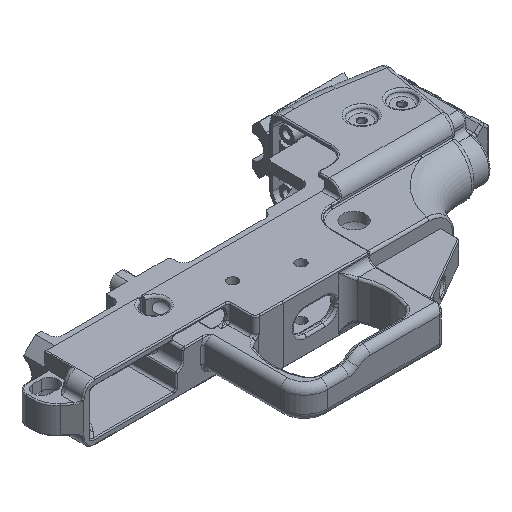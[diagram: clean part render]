
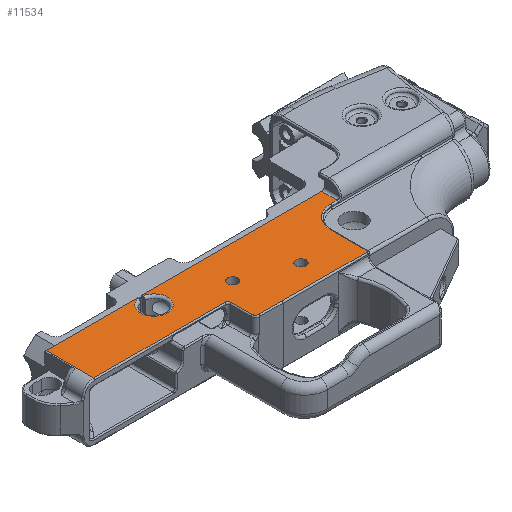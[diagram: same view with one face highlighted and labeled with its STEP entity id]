
A CAD part, isometric view. The second image highlights one B-rep face of the part: STEP entity #11534.
In plain terms, the highlighted face is planar.
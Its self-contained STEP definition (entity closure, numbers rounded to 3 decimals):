
#192=FACE_BOUND('',#2251,.T.);
#193=FACE_BOUND('',#2252,.T.);
#549=CIRCLE('',#12264,2.175);
#551=CIRCLE('',#12267,2.175);
#599=CIRCLE('',#12346,5.875);
#602=CIRCLE('',#12353,0.5);
#605=CIRCLE('',#12357,0.5);
#609=CIRCLE('',#12363,1.5);
#610=CIRCLE('',#12364,1.5);
#611=CIRCLE('',#12365,0.5);
#612=CIRCLE('',#12366,9.5);
#1534=FACE_OUTER_BOUND('',#2250,.T.);
#2250=EDGE_LOOP('',(#7943,#7944,#7945,#7946,#7947,#7948,#7949,#7950,#7951,
#7952,#7953,#7954,#7955,#7956,#7957,#7958,#7959,#7960,#7961));
#2251=EDGE_LOOP('',(#7962));
#2252=EDGE_LOOP('',(#7963));
#2956=LINE('',#17332,#3840);
#2996=LINE('',#17995,#3880);
#3036=LINE('',#18155,#3920);
#3038=LINE('',#18324,#3922);
#3046=LINE('',#18387,#3930);
#3047=LINE('',#18389,#3931);
#3048=LINE('',#18393,#3932);
#3049=LINE('',#18397,#3933);
#3050=LINE('',#18399,#3934);
#3051=LINE('',#18403,#3935);
#3052=LINE('',#18407,#3936);
#3053=LINE('',#18408,#3937);
#3840=VECTOR('',#13659,10.);
#3880=VECTOR('',#13839,10.);
#3920=VECTOR('',#13969,10.);
#3922=VECTOR('',#13977,10.);
#3930=VECTOR('',#14007,39.75);
#3931=VECTOR('',#14008,10.);
#3932=VECTOR('',#14011,10.);
#3933=VECTOR('',#14014,10.);
#3934=VECTOR('',#14015,10.);
#3935=VECTOR('',#14018,10.);
#3936=VECTOR('',#14021,10.);
#3937=VECTOR('',#14022,10.);
#4730=VERTEX_POINT('',#17329);
#4731=VERTEX_POINT('',#17331);
#4769=VERTEX_POINT('',#17462);
#4771=VERTEX_POINT('',#17468);
#4810=VERTEX_POINT('',#17992);
#4811=VERTEX_POINT('',#17994);
#4861=VERTEX_POINT('',#18122);
#4862=VERTEX_POINT('',#18133);
#4866=VERTEX_POINT('',#18153);
#4873=VERTEX_POINT('',#18323);
#4878=VERTEX_POINT('',#18338);
#4884=VERTEX_POINT('',#18388);
#4885=VERTEX_POINT('',#18390);
#4886=VERTEX_POINT('',#18392);
#4887=VERTEX_POINT('',#18394);
#4888=VERTEX_POINT('',#18396);
#4889=VERTEX_POINT('',#18398);
#4890=VERTEX_POINT('',#18400);
#4891=VERTEX_POINT('',#18402);
#4892=VERTEX_POINT('',#18404);
#4893=VERTEX_POINT('',#18406);
#5839=EDGE_CURVE('',#4730,#4731,#2956,.T.);
#5887=EDGE_CURVE('',#4769,#4769,#549,.T.);
#5890=EDGE_CURVE('',#4771,#4771,#551,.T.);
#5945=EDGE_CURVE('',#4810,#4811,#2996,.T.);
#6009=EDGE_CURVE('',#4861,#4862,#599,.T.);
#6016=EDGE_CURVE('',#4861,#4866,#3036,.T.);
#6025=EDGE_CURVE('',#4873,#4862,#3038,.T.);
#6029=EDGE_CURVE('',#4730,#4873,#602,.T.);
#6033=EDGE_CURVE('',#4866,#4878,#605,.T.);
#6041=EDGE_CURVE('',#4811,#4878,#3046,.T.);
#6042=EDGE_CURVE('',#4884,#4810,#3047,.T.);
#6043=EDGE_CURVE('',#4885,#4884,#609,.T.);
#6044=EDGE_CURVE('',#4886,#4885,#3048,.T.);
#6045=EDGE_CURVE('',#4887,#4886,#610,.T.);
#6046=EDGE_CURVE('',#4888,#4887,#3049,.T.);
#6047=EDGE_CURVE('',#4889,#4888,#3050,.T.);
#6048=EDGE_CURVE('',#4890,#4889,#611,.T.);
#6049=EDGE_CURVE('',#4891,#4890,#3051,.T.);
#6050=EDGE_CURVE('',#4892,#4891,#612,.T.);
#6051=EDGE_CURVE('',#4893,#4892,#3052,.T.);
#6052=EDGE_CURVE('',#4731,#4893,#3053,.T.);
#7943=ORIENTED_EDGE('',*,*,#6041,.F.);
#7944=ORIENTED_EDGE('',*,*,#5945,.F.);
#7945=ORIENTED_EDGE('',*,*,#6042,.F.);
#7946=ORIENTED_EDGE('',*,*,#6043,.F.);
#7947=ORIENTED_EDGE('',*,*,#6044,.F.);
#7948=ORIENTED_EDGE('',*,*,#6045,.F.);
#7949=ORIENTED_EDGE('',*,*,#6046,.F.);
#7950=ORIENTED_EDGE('',*,*,#6047,.F.);
#7951=ORIENTED_EDGE('',*,*,#6048,.F.);
#7952=ORIENTED_EDGE('',*,*,#6049,.F.);
#7953=ORIENTED_EDGE('',*,*,#6050,.F.);
#7954=ORIENTED_EDGE('',*,*,#6051,.F.);
#7955=ORIENTED_EDGE('',*,*,#6052,.F.);
#7956=ORIENTED_EDGE('',*,*,#5839,.F.);
#7957=ORIENTED_EDGE('',*,*,#6029,.T.);
#7958=ORIENTED_EDGE('',*,*,#6025,.T.);
#7959=ORIENTED_EDGE('',*,*,#6009,.F.);
#7960=ORIENTED_EDGE('',*,*,#6016,.T.);
#7961=ORIENTED_EDGE('',*,*,#6033,.T.);
#7962=ORIENTED_EDGE('',*,*,#5890,.T.);
#7963=ORIENTED_EDGE('',*,*,#5887,.T.);
#11255=PLANE('',#12362);
#11534=ADVANCED_FACE('',(#1534,#192,#193),#11255,.T.);
#12264=AXIS2_PLACEMENT_3D('',#17463,#13744,#13745);
#12267=AXIS2_PLACEMENT_3D('',#17469,#13751,#13752);
#12346=AXIS2_PLACEMENT_3D('',#18134,#13959,#13960);
#12353=AXIS2_PLACEMENT_3D('',#18331,#13983,#13984);
#12357=AXIS2_PLACEMENT_3D('',#18339,#13992,#13993);
#12362=AXIS2_PLACEMENT_3D('',#18386,#14005,#14006);
#12363=AXIS2_PLACEMENT_3D('',#18391,#14009,#14010);
#12364=AXIS2_PLACEMENT_3D('',#18395,#14012,#14013);
#12365=AXIS2_PLACEMENT_3D('',#18401,#14016,#14017);
#12366=AXIS2_PLACEMENT_3D('',#18405,#14019,#14020);
#13659=DIRECTION('',(-1.,0.,0.));
#13744=DIRECTION('center_axis',(0.,0.,1.));
#13745=DIRECTION('ref_axis',(1.,0.,0.));
#13751=DIRECTION('center_axis',(0.,0.,1.));
#13752=DIRECTION('ref_axis',(1.,0.,0.));
#13839=DIRECTION('',(0.,1.,0.));
#13959=DIRECTION('center_axis',(0.,0.,-1.));
#13960=DIRECTION('ref_axis',(0.,-1.,0.));
#13969=DIRECTION('',(0.,1.,0.));
#13977=DIRECTION('',(0.,-1.,0.));
#13983=DIRECTION('center_axis',(0.,0.,1.));
#13984=DIRECTION('ref_axis',(-0.707,0.707,0.));
#13992=DIRECTION('center_axis',(0.,0.,1.));
#13993=DIRECTION('ref_axis',(0.707,0.707,0.));
#14005=DIRECTION('center_axis',(0.,0.,-1.));
#14006=DIRECTION('ref_axis',(1.,0.,0.));
#14007=DIRECTION('',(-1.,0.,0.));
#14008=DIRECTION('',(1.,0.,0.));
#14009=DIRECTION('center_axis',(0.,0.,-1.));
#14010=DIRECTION('ref_axis',(-0.707,0.707,0.));
#14011=DIRECTION('',(0.,1.,0.));
#14012=DIRECTION('center_axis',(0.,0.,1.));
#14013=DIRECTION('ref_axis',(0.71,-0.704,0.));
#14014=DIRECTION('',(1.,0.008,0.));
#14015=DIRECTION('',(1.,0.,0.));
#14016=DIRECTION('center_axis',(0.,0.,1.));
#14017=DIRECTION('ref_axis',(-0.707,-0.707,0.));
#14018=DIRECTION('',(0.,-1.,0.));
#14019=DIRECTION('center_axis',(0.,0.,-1.));
#14020=DIRECTION('ref_axis',(0.707,0.707,0.));
#14021=DIRECTION('',(1.,0.,0.));
#14022=DIRECTION('',(0.,-1.,0.));
#17329=CARTESIAN_POINT('',(111.061,21.019,-12.457));
#17331=CARTESIAN_POINT('',(33.41,21.019,-12.457));
#17332=CARTESIAN_POINT('',(81.026,21.019,-12.457));
#17462=CARTESIAN_POINT('',(62.366,-1.177,-12.457));
#17463=CARTESIAN_POINT('Origin',(64.541,-1.177,-12.457));
#17468=CARTESIAN_POINT('',(83.779,6.799,-12.457));
#17469=CARTESIAN_POINT('Origin',(85.954,6.799,-12.457));
#17992=CARTESIAN_POINT('',(152.201,0.5,-12.457));
#17994=CARTESIAN_POINT('',(152.201,21.019,-12.457));
#17995=CARTESIAN_POINT('',(152.201,-48.911,-12.457));
#18122=CARTESIAN_POINT('',(112.98,20.523,-12.457));
#18133=CARTESIAN_POINT('',(110.999,20.523,-12.457));
#18134=CARTESIAN_POINT('Origin',(111.989,14.732,-12.457));
#18153=CARTESIAN_POINT('',(112.98,20.776,-12.457));
#18155=CARTESIAN_POINT('',(112.98,-44.635,-12.457));
#18323=CARTESIAN_POINT('',(110.999,20.776,-12.457));
#18324=CARTESIAN_POINT('',(110.999,-43.582,-12.457));
#18331=CARTESIAN_POINT('Origin',(111.499,20.776,-12.457));
#18338=CARTESIAN_POINT('',(112.917,21.019,-12.457));
#18339=CARTESIAN_POINT('Origin',(112.48,20.776,-12.457));
#18386=CARTESIAN_POINT('Origin',(83.274,-108.44,-12.457));
#18387=CARTESIAN_POINT('',(152.73,21.019,-12.457));
#18388=CARTESIAN_POINT('',(95.882,0.5,-12.457));
#18389=CARTESIAN_POINT('',(41.637,0.5,-12.457));
#18390=CARTESIAN_POINT('',(94.382,-1.,-12.457));
#18391=CARTESIAN_POINT('Origin',(95.882,-1.,-12.457));
#18392=CARTESIAN_POINT('',(94.382,-9.796,-12.457));
#18393=CARTESIAN_POINT('',(94.382,-54.22,-12.457));
#18394=CARTESIAN_POINT('',(92.893,-11.296,-12.457));
#18395=CARTESIAN_POINT('Origin',(92.882,-9.796,-12.457));
#18396=CARTESIAN_POINT('',(83.007,-11.373,-12.457));
#18397=CARTESIAN_POINT('',(82.761,-11.375,-12.457));
#18398=CARTESIAN_POINT('',(46.306,-11.373,-12.457));
#18399=CARTESIAN_POINT('',(83.141,-11.373,-12.457));
#18400=CARTESIAN_POINT('',(45.806,-10.873,-12.457));
#18401=CARTESIAN_POINT('Origin',(46.306,-10.873,-12.457));
#18402=CARTESIAN_POINT('',(45.806,4.878,-12.457));
#18403=CARTESIAN_POINT('',(45.806,-60.157,-12.457));
#18404=CARTESIAN_POINT('',(36.306,14.378,-12.457));
#18405=CARTESIAN_POINT('Origin',(36.306,4.878,-12.457));
#18406=CARTESIAN_POINT('',(33.41,14.378,-12.457));
#18407=CARTESIAN_POINT('',(44.137,14.378,-12.457));
#18408=CARTESIAN_POINT('',(33.41,-108.44,-12.457));
